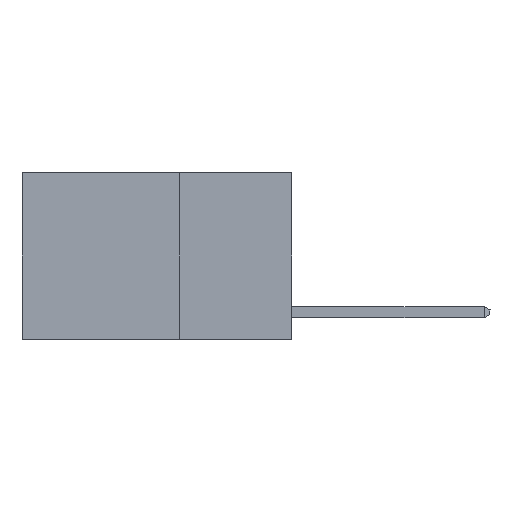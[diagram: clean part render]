
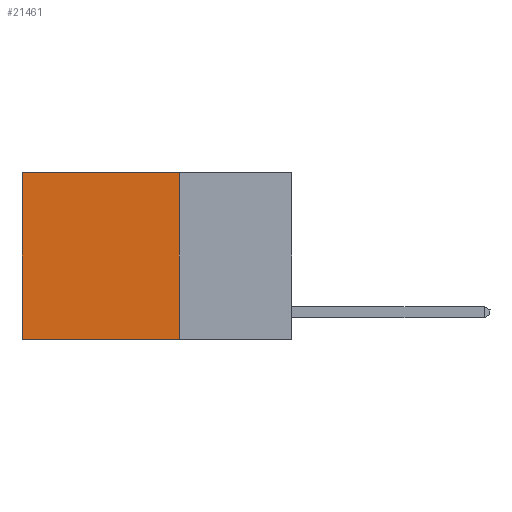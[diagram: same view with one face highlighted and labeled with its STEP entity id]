
A CAD part, left-side view. The second image highlights one B-rep face of the part: STEP entity #21461.
In plain terms, the highlighted planar face has unit normal (-1, 0, 0).
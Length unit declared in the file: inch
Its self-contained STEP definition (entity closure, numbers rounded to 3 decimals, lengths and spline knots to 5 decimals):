
#501 = AXIS2_PLACEMENT_3D ( 'NONE', #7760, #13511, #2140 ) ;
#1462 = LINE ( 'NONE', #22196, #10940 ) ;
#2065 = EDGE_CURVE ( 'NONE', #18628, #14685, #13741, .T. ) ;
#2140 = DIRECTION ( 'NONE',  ( 0., 0., -1. ) ) ;
#2350 = ORIENTED_EDGE ( 'NONE', *, *, #5656, .F. ) ;
#4433 = CARTESIAN_POINT ( 'NONE',  ( 0.2625, 0.25, 0. ) ) ;
#5656 = EDGE_CURVE ( 'NONE', #14989, #13430, #9332, .T. ) ;
#6856 = CARTESIAN_POINT ( 'NONE',  ( 0.2625, 0.25, -0.37 ) ) ;
#7760 = CARTESIAN_POINT ( 'NONE',  ( 0.2625, 0.25, 0. ) ) ;
#9032 = DIRECTION ( 'NONE',  ( 0., 1., 0. ) ) ;
#9332 = LINE ( 'NONE', #12928, #18797 ) ;
#9395 = CARTESIAN_POINT ( 'NONE',  ( 0.2625, 0.6, 0. ) ) ;
#10029 = CARTESIAN_POINT ( 'NONE',  ( 0.2625, 0.25, 0. ) ) ;
#10940 = VECTOR ( 'NONE', #9032, 39.37008 ) ;
#11315 = DIRECTION ( 'NONE',  ( 0., 0., -1. ) ) ;
#11553 = FACE_OUTER_BOUND ( 'NONE', #18860, .T. ) ;
#12649 = ORIENTED_EDGE ( 'NONE', *, *, #23853, .T. ) ;
#12928 = CARTESIAN_POINT ( 'NONE',  ( 0.2625, 0.25, 0. ) ) ;
#13430 = VERTEX_POINT ( 'NONE', #6856 ) ;
#13511 = DIRECTION ( 'NONE',  ( 1., 0., 0. ) ) ;
#13724 = ORIENTED_EDGE ( 'NONE', *, *, #2065, .T. ) ;
#13741 = LINE ( 'NONE', #9395, #18678 ) ;
#14685 = VERTEX_POINT ( 'NONE', #16367 ) ;
#14989 = VERTEX_POINT ( 'NONE', #10029 ) ;
#16367 = CARTESIAN_POINT ( 'NONE',  ( 0.2625, 0.6, -0.37 ) ) ;
#16615 = EDGE_CURVE ( 'NONE', #13430, #14685, #1462, .T. ) ;
#17158 = CARTESIAN_POINT ( 'NONE',  ( 0.2625, 0.6, 0. ) ) ;
#17194 = PLANE ( 'NONE',  #501 ) ;
#18628 = VERTEX_POINT ( 'NONE', #17158 ) ;
#18678 = VECTOR ( 'NONE', #11315, 39.37008 ) ;
#18797 = VECTOR ( 'NONE', #20417, 39.37008 ) ;
#18860 = EDGE_LOOP ( 'NONE', ( #13724, #19088, #2350, #12649 ) ) ;
#19088 = ORIENTED_EDGE ( 'NONE', *, *, #16615, .F. ) ;
#19512 = DIRECTION ( 'NONE',  ( 0., 1., 0. ) ) ;
#20417 = DIRECTION ( 'NONE',  ( 0., 0., -1. ) ) ;
#21461 = ADVANCED_FACE ( 'NONE', ( #11553 ), #17194, .F. ) ;
#22196 = CARTESIAN_POINT ( 'NONE',  ( 0.2625, 0.25, -0.37 ) ) ;
#22301 = VECTOR ( 'NONE', #19512, 39.37008 ) ;
#22886 = LINE ( 'NONE', #4433, #22301 ) ;
#23853 = EDGE_CURVE ( 'NONE', #14989, #18628, #22886, .T. ) ;
